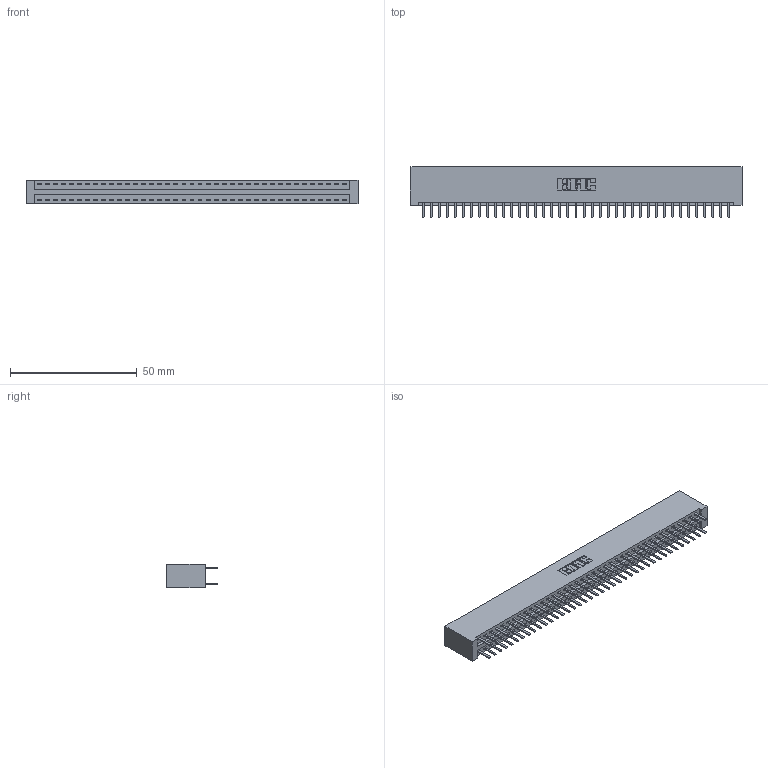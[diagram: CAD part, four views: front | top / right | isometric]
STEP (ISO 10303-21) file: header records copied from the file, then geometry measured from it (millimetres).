
FILE_DESCRIPTION (( 'STEP AP203' ), '1' );
FILE_NAME ('396-078-520-201.STEP', '2019-10-30T21:45:33', ( '' ), ( '' ), 'SwSTEP 2.0', 'SolidWorks 2016', '' );
FILE_SCHEMA (( 'CONFIG_CONTROL_DESIGN' ));
Length unit declared in the file: inch
Products named in the file (3): 345-292-001_345-293-120; 346 Part_No Mounting Lugs; 396-078-520-201
Assembly tree (79 placements, depth 2):
  396-078-520-201
    346 Part_No Mounting Lugs
    345-292-001_345-293-120  x78
Bounding box: 131.06 x 20.02 x 9.4 mm (x, y, z)
Volume: 13296.1 mm3; surface area: 18312 mm2
Topology: 79 solids, 79 shells, 4482 faces, 13019 edges, 8470 vertices
Faces by surface type: plane 2958, cylinder 1524
Entity records: 25693 total; most frequent: CARTESIAN_POINT 4248, ORIENTED_EDGE 4170, DIRECTION 3777, EDGE_CURVE 2085, VECTOR 1801, LINE 1801, VERTEX_POINT 1386, AXIS2_PLACEMENT_3D 988
